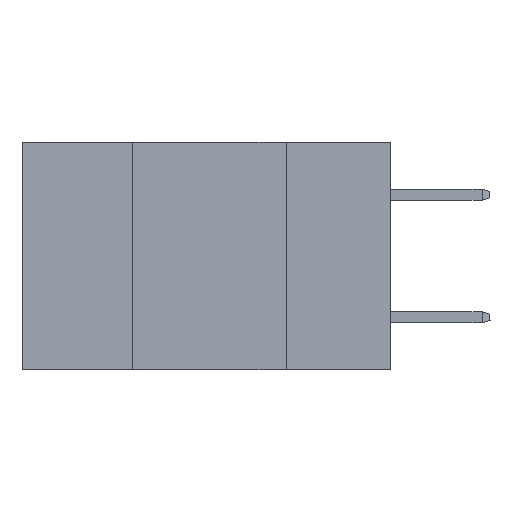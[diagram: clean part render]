
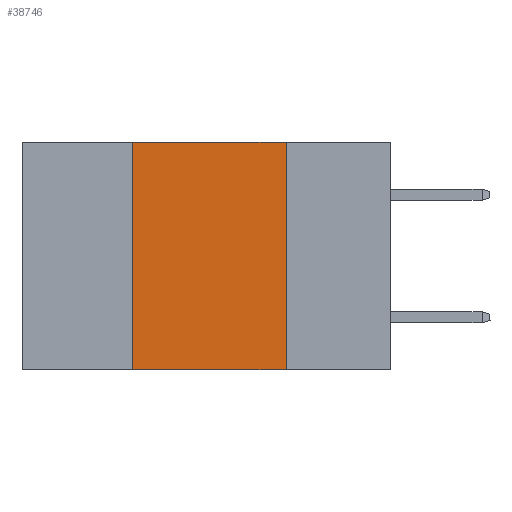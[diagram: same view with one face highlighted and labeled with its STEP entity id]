
A CAD part, left-side view. The second image highlights one B-rep face of the part: STEP entity #38746.
In plain terms, the highlighted planar face has unit normal (-1, 0, 0).
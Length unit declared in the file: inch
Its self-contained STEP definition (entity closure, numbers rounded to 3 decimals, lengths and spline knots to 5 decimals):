
#353 = ORIENTED_EDGE ( 'NONE', *, *, #20929, .F. ) ;
#406 = DIRECTION ( 'NONE',  ( 0., -1., 0. ) ) ;
#3581 = VECTOR ( 'NONE', #37411, 39.37008 ) ;
#4778 = CARTESIAN_POINT ( 'NONE',  ( 0., 0.42, 0. ) ) ;
#5309 = DIRECTION ( 'NONE',  ( 0., 0., -1. ) ) ;
#7980 = LINE ( 'NONE', #16237, #30125 ) ;
#8026 = VERTEX_POINT ( 'NONE', #13294 ) ;
#10852 = ORIENTED_EDGE ( 'NONE', *, *, #25832, .F. ) ;
#10970 = ORIENTED_EDGE ( 'NONE', *, *, #22978, .F. ) ;
#11793 = CARTESIAN_POINT ( 'NONE',  ( 0., 0.17, 0. ) ) ;
#13294 = CARTESIAN_POINT ( 'NONE',  ( 0., 0.42, -0.37 ) ) ;
#15472 = VERTEX_POINT ( 'NONE', #4778 ) ;
#16237 = CARTESIAN_POINT ( 'NONE',  ( 0., 0.42, 0. ) ) ;
#17498 = DIRECTION ( 'NONE',  ( 0., 0., -1. ) ) ;
#18487 = EDGE_LOOP ( 'NONE', ( #353, #10852, #10970, #20907 ) ) ;
#19198 = VERTEX_POINT ( 'NONE', #29069 ) ;
#19962 = DIRECTION ( 'NONE',  ( 0., 0., 1. ) ) ;
#20239 = DIRECTION ( 'NONE',  ( 1., 0., 0. ) ) ;
#20907 = ORIENTED_EDGE ( 'NONE', *, *, #32730, .T. ) ;
#20929 = EDGE_CURVE ( 'NONE', #29889, #19198, #30057, .T. ) ;
#21244 = AXIS2_PLACEMENT_3D ( 'NONE', #32609, #20239, #5309 ) ;
#21438 = LINE ( 'NONE', #36170, #37802 ) ;
#22978 = EDGE_CURVE ( 'NONE', #8026, #15472, #7980, .T. ) ;
#25832 = EDGE_CURVE ( 'NONE', #15472, #29889, #21438, .T. ) ;
#26357 = VECTOR ( 'NONE', #17498, 39.37008 ) ;
#28566 = LINE ( 'NONE', #31713, #3581 ) ;
#29069 = CARTESIAN_POINT ( 'NONE',  ( 0., 0.17, -0.37 ) ) ;
#29261 = FACE_OUTER_BOUND ( 'NONE', #18487, .T. ) ;
#29889 = VERTEX_POINT ( 'NONE', #34361 ) ;
#30057 = LINE ( 'NONE', #11793, #26357 ) ;
#30125 = VECTOR ( 'NONE', #19962, 39.37008 ) ;
#31713 = CARTESIAN_POINT ( 'NONE',  ( 0., 0.6, -0.37 ) ) ;
#32609 = CARTESIAN_POINT ( 'NONE',  ( 0., 0.6, 0. ) ) ;
#32730 = EDGE_CURVE ( 'NONE', #8026, #19198, #28566, .T. ) ;
#34361 = CARTESIAN_POINT ( 'NONE',  ( 0., 0.17, 0. ) ) ;
#36170 = CARTESIAN_POINT ( 'NONE',  ( 0., 0.6, 0. ) ) ;
#37411 = DIRECTION ( 'NONE',  ( 0., -1., 0. ) ) ;
#37802 = VECTOR ( 'NONE', #406, 39.37008 ) ;
#38301 = PLANE ( 'NONE',  #21244 ) ;
#38746 = ADVANCED_FACE ( 'NONE', ( #29261 ), #38301, .F. ) ;
